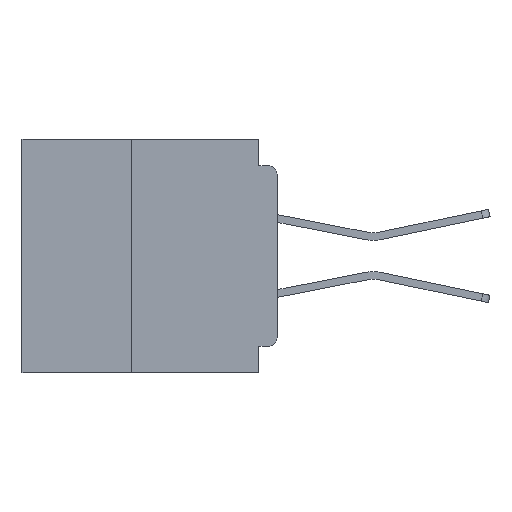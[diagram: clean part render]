
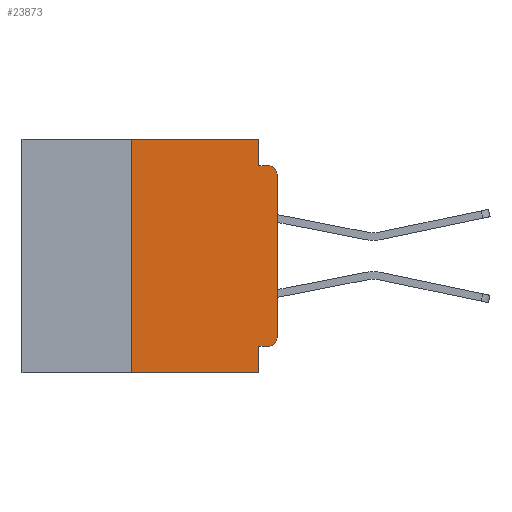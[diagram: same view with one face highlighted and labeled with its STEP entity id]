
A CAD part, left-side view. The second image highlights one B-rep face of the part: STEP entity #23873.
In plain terms, the highlighted planar face has unit normal (-1, 0, 0).
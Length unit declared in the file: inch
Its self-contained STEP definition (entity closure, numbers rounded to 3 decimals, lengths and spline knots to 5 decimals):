
#621 = AXIS2_PLACEMENT_3D ( 'NONE', #16837, #1477, #22937 ) ;
#973 = VECTOR ( 'NONE', #23311, 39.37008 ) ;
#1477 = DIRECTION ( 'NONE',  ( 1., 0., 0. ) ) ;
#2468 = VECTOR ( 'NONE', #21193, 39.37008 ) ;
#2651 = DIRECTION ( 'NONE',  ( 0., 0., 1. ) ) ;
#2914 = CARTESIAN_POINT ( 'NONE',  ( 0., 0.031, -0.4 ) ) ;
#2924 = EDGE_CURVE ( 'NONE', #12927, #28644, #10581, .T. ) ;
#3212 = CARTESIAN_POINT ( 'NONE',  ( 0., 0., -0.06 ) ) ;
#3251 = CARTESIAN_POINT ( 'NONE',  ( 0., 0.031, 0. ) ) ;
#4767 = ORIENTED_EDGE ( 'NONE', *, *, #27769, .T. ) ;
#6213 = VECTOR ( 'NONE', #2651, 39.37008 ) ;
#6262 = VECTOR ( 'NONE', #22518, 39.37008 ) ;
#6385 = DIRECTION ( 'NONE',  ( 0., 0., -1. ) ) ;
#7816 = CARTESIAN_POINT ( 'NONE',  ( 0., 0.031, -0.4 ) ) ;
#8254 = VERTEX_POINT ( 'NONE', #2914 ) ;
#8673 = CARTESIAN_POINT ( 'NONE',  ( 0., 0.25, -0.4 ) ) ;
#8936 = LINE ( 'NONE', #3251, #32069 ) ;
#9270 = LINE ( 'NONE', #38126, #973 ) ;
#9459 = ORIENTED_EDGE ( 'NONE', *, *, #20151, .T. ) ;
#9516 = ORIENTED_EDGE ( 'NONE', *, *, #37048, .F. ) ;
#10581 = CIRCLE ( 'NONE', #16480, 0.015 ) ;
#11138 = ORIENTED_EDGE ( 'NONE', *, *, #2924, .T. ) ;
#11575 = VERTEX_POINT ( 'NONE', #12223 ) ;
#12223 = CARTESIAN_POINT ( 'NONE',  ( 0., 0.25, 0. ) ) ;
#12316 = VERTEX_POINT ( 'NONE', #30473 ) ;
#12521 = EDGE_CURVE ( 'NONE', #15736, #29249, #15371, .T. ) ;
#12927 = VERTEX_POINT ( 'NONE', #3212 ) ;
#13355 = CARTESIAN_POINT ( 'NONE',  ( 0., 0., -0.355 ) ) ;
#13555 = EDGE_CURVE ( 'NONE', #18838, #28644, #30789, .T. ) ;
#14378 = LINE ( 'NONE', #27017, #6213 ) ;
#14550 = LINE ( 'NONE', #7816, #30529 ) ;
#14556 = CARTESIAN_POINT ( 'NONE',  ( 0., 0.437, 0. ) ) ;
#14808 = VECTOR ( 'NONE', #29660, 39.37008 ) ;
#15371 = LINE ( 'NONE', #13355, #6262 ) ;
#15736 = VERTEX_POINT ( 'NONE', #24280 ) ;
#16063 = DIRECTION ( 'NONE',  ( -1., 0., 0. ) ) ;
#16268 = CIRCLE ( 'NONE', #34167, 0.015 ) ;
#16398 = CARTESIAN_POINT ( 'NONE',  ( 0., 0.031, -0.045 ) ) ;
#16480 = AXIS2_PLACEMENT_3D ( 'NONE', #16925, #16698, #16572 ) ;
#16542 = EDGE_LOOP ( 'NONE', ( #37722, #11138, #21943, #21262, #24183, #9516, #4767, #18158, #17507, #9459 ) ) ;
#16572 = DIRECTION ( 'NONE',  ( 0., 0., -1. ) ) ;
#16698 = DIRECTION ( 'NONE',  ( -1., 0., 0. ) ) ;
#16837 = CARTESIAN_POINT ( 'NONE',  ( 0., 0.437, 0. ) ) ;
#16925 = CARTESIAN_POINT ( 'NONE',  ( 0., 0.015, -0.06 ) ) ;
#17507 = ORIENTED_EDGE ( 'NONE', *, *, #12521, .F. ) ;
#17737 = EDGE_CURVE ( 'NONE', #29249, #8254, #14550, .T. ) ;
#18158 = ORIENTED_EDGE ( 'NONE', *, *, #17737, .F. ) ;
#18525 = EDGE_CURVE ( 'NONE', #23502, #12927, #18829, .T. ) ;
#18829 = LINE ( 'NONE', #30079, #2468 ) ;
#18838 = VERTEX_POINT ( 'NONE', #16398 ) ;
#20151 = EDGE_CURVE ( 'NONE', #15736, #23502, #16268, .T. ) ;
#21193 = DIRECTION ( 'NONE',  ( 0., 0., 1. ) ) ;
#21262 = ORIENTED_EDGE ( 'NONE', *, *, #22318, .F. ) ;
#21943 = ORIENTED_EDGE ( 'NONE', *, *, #13555, .F. ) ;
#22318 = EDGE_CURVE ( 'NONE', #12316, #18838, #8936, .T. ) ;
#22518 = DIRECTION ( 'NONE',  ( 0., 1., 0. ) ) ;
#22577 = LINE ( 'NONE', #14556, #37484 ) ;
#22764 = VERTEX_POINT ( 'NONE', #8673 ) ;
#22937 = DIRECTION ( 'NONE',  ( 0., 0., -1. ) ) ;
#23311 = DIRECTION ( 'NONE',  ( 0., -1., 0. ) ) ;
#23502 = VERTEX_POINT ( 'NONE', #36116 ) ;
#23873 = ADVANCED_FACE ( 'NONE', ( #31242 ), #34795, .F. ) ;
#24183 = ORIENTED_EDGE ( 'NONE', *, *, #27844, .F. ) ;
#24280 = CARTESIAN_POINT ( 'NONE',  ( 0., 0.015, -0.355 ) ) ;
#27017 = CARTESIAN_POINT ( 'NONE',  ( 0., 0.25, -0.4 ) ) ;
#27769 = EDGE_CURVE ( 'NONE', #22764, #8254, #9270, .T. ) ;
#27844 = EDGE_CURVE ( 'NONE', #11575, #12316, #22577, .T. ) ;
#28644 = VERTEX_POINT ( 'NONE', #37878 ) ;
#28955 = DIRECTION ( 'NONE',  ( 0., 0., -1. ) ) ;
#29249 = VERTEX_POINT ( 'NONE', #34617 ) ;
#29660 = DIRECTION ( 'NONE',  ( 0., -1., 0. ) ) ;
#30079 = CARTESIAN_POINT ( 'NONE',  ( 0., 0., 0. ) ) ;
#30473 = CARTESIAN_POINT ( 'NONE',  ( 0., 0.031, 0. ) ) ;
#30529 = VECTOR ( 'NONE', #28955, 39.37008 ) ;
#30789 = LINE ( 'NONE', #32555, #14808 ) ;
#31242 = FACE_OUTER_BOUND ( 'NONE', #16542, .T. ) ;
#32069 = VECTOR ( 'NONE', #6385, 39.37008 ) ;
#32555 = CARTESIAN_POINT ( 'NONE',  ( 0., 0., -0.045 ) ) ;
#32588 = DIRECTION ( 'NONE',  ( 0., -1., 0. ) ) ;
#34055 = CARTESIAN_POINT ( 'NONE',  ( 0., 0.015, -0.34 ) ) ;
#34167 = AXIS2_PLACEMENT_3D ( 'NONE', #34055, #16063, #37033 ) ;
#34617 = CARTESIAN_POINT ( 'NONE',  ( 0., 0.031, -0.355 ) ) ;
#34795 = PLANE ( 'NONE',  #621 ) ;
#36116 = CARTESIAN_POINT ( 'NONE',  ( 0., 0., -0.34 ) ) ;
#37033 = DIRECTION ( 'NONE',  ( 0., 0., -1. ) ) ;
#37048 = EDGE_CURVE ( 'NONE', #22764, #11575, #14378, .T. ) ;
#37484 = VECTOR ( 'NONE', #32588, 39.37008 ) ;
#37722 = ORIENTED_EDGE ( 'NONE', *, *, #18525, .T. ) ;
#37878 = CARTESIAN_POINT ( 'NONE',  ( 0., 0.015, -0.045 ) ) ;
#38126 = CARTESIAN_POINT ( 'NONE',  ( 0., 0.437, -0.4 ) ) ;
